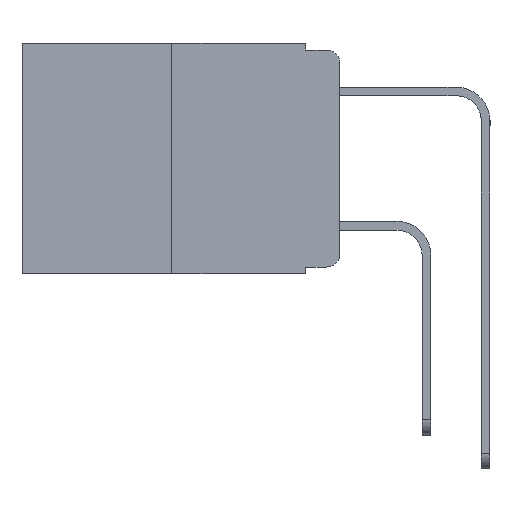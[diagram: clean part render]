
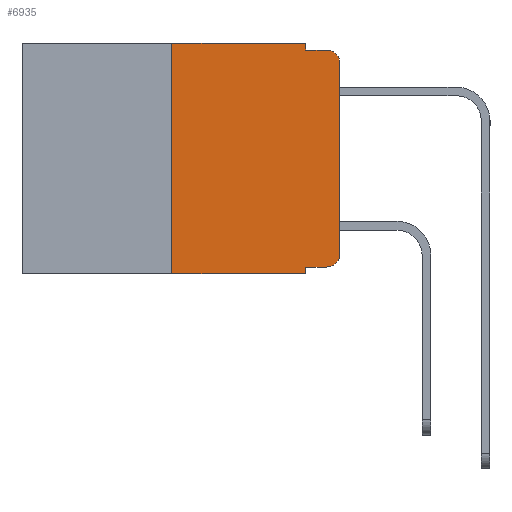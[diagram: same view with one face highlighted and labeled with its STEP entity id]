
A CAD part, left-side view. The second image highlights one B-rep face of the part: STEP entity #6935.
In plain terms, the highlighted planar face has unit normal (-1, 0, 0).
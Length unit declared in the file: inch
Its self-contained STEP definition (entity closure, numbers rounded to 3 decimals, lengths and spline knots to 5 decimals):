
#8 = FACE_OUTER_BOUND ( 'NONE', #3519, .T. ) ;
#575 = LINE ( 'NONE', #6948, #2765 ) ;
#703 = VECTOR ( 'NONE', #7074, 39.37008 ) ;
#1054 = CIRCLE ( 'NONE', #3146, 0.02 ) ;
#1242 = CARTESIAN_POINT ( 'NONE',  ( 0., 0.473, -0.343 ) ) ;
#1650 = CARTESIAN_POINT ( 'NONE',  ( 0., 0.02, -0.333 ) ) ;
#1763 = DIRECTION ( 'NONE',  ( 0., -1., 0. ) ) ;
#1765 = DIRECTION ( 'NONE',  ( 0., 0., 1. ) ) ;
#1862 = LINE ( 'NONE', #2055, #4319 ) ;
#2035 = VERTEX_POINT ( 'NONE', #3989 ) ;
#2053 = CARTESIAN_POINT ( 'NONE',  ( 0., 0.051, -0.333 ) ) ;
#2055 = CARTESIAN_POINT ( 'NONE',  ( 0., 0.051, 0. ) ) ;
#2287 = ORIENTED_EDGE ( 'NONE', *, *, #8767, .F. ) ;
#2603 = EDGE_CURVE ( 'NONE', #3111, #4419, #6063, .T. ) ;
#2765 = VECTOR ( 'NONE', #3821, 39.37008 ) ;
#2806 = ORIENTED_EDGE ( 'NONE', *, *, #2603, .T. ) ;
#2882 = CARTESIAN_POINT ( 'NONE',  ( 0., 0.02, -0.01 ) ) ;
#2961 = CARTESIAN_POINT ( 'NONE',  ( 0., 0.25, 0. ) ) ;
#3032 = DIRECTION ( 'NONE',  ( 0., -1., 0. ) ) ;
#3111 = VERTEX_POINT ( 'NONE', #1650 ) ;
#3146 = AXIS2_PLACEMENT_3D ( 'NONE', #10799, #4882, #11763 ) ;
#3317 = EDGE_CURVE ( 'NONE', #5770, #3111, #3462, .T. ) ;
#3462 = LINE ( 'NONE', #2053, #8555 ) ;
#3519 = EDGE_LOOP ( 'NONE', ( #10459, #9419, #2287, #11503, #12666, #12368, #8058, #8974, #6822, #2806 ) ) ;
#3821 = DIRECTION ( 'NONE',  ( 0., -1., 0. ) ) ;
#3989 = CARTESIAN_POINT ( 'NONE',  ( 0., 0., -0.03 ) ) ;
#4093 = CARTESIAN_POINT ( 'NONE',  ( 0., 0.051, -0.01 ) ) ;
#4191 = EDGE_CURVE ( 'NONE', #12171, #9761, #7765, .T. ) ;
#4319 = VECTOR ( 'NONE', #12962, 39.37008 ) ;
#4419 = VERTEX_POINT ( 'NONE', #6970 ) ;
#4425 = PLANE ( 'NONE',  #4759 ) ;
#4682 = CARTESIAN_POINT ( 'NONE',  ( 0., 0.051, -0.333 ) ) ;
#4699 = EDGE_CURVE ( 'NONE', #5770, #9761, #8820, .T. ) ;
#4759 = AXIS2_PLACEMENT_3D ( 'NONE', #11334, #5464, #12274 ) ;
#4882 = DIRECTION ( 'NONE',  ( -1., 0., 0. ) ) ;
#5383 = EDGE_CURVE ( 'NONE', #12171, #12336, #6310, .T. ) ;
#5464 = DIRECTION ( 'NONE',  ( 1., 0., 0. ) ) ;
#5770 = VERTEX_POINT ( 'NONE', #4682 ) ;
#6063 = CIRCLE ( 'NONE', #12346, 0.02 ) ;
#6310 = LINE ( 'NONE', #2961, #703 ) ;
#6785 = EDGE_CURVE ( 'NONE', #10905, #12877, #1862, .T. ) ;
#6822 = ORIENTED_EDGE ( 'NONE', *, *, #3317, .T. ) ;
#6844 = CARTESIAN_POINT ( 'NONE',  ( 0., 0.051, 0. ) ) ;
#6906 = CARTESIAN_POINT ( 'NONE',  ( 0., 0.473, 0. ) ) ;
#6935 = ADVANCED_FACE ( 'NONE', ( #8 ), #4425, .F. ) ;
#6948 = CARTESIAN_POINT ( 'NONE',  ( 0., 0.051, -0.01 ) ) ;
#6961 = CARTESIAN_POINT ( 'NONE',  ( 0., 0., 0. ) ) ;
#6970 = CARTESIAN_POINT ( 'NONE',  ( 0., 0., -0.313 ) ) ;
#7074 = DIRECTION ( 'NONE',  ( 0., 0., 1. ) ) ;
#7094 = LINE ( 'NONE', #6961, #7417 ) ;
#7115 = EDGE_CURVE ( 'NONE', #12336, #10905, #11371, .T. ) ;
#7417 = VECTOR ( 'NONE', #1765, 39.37008 ) ;
#7456 = VECTOR ( 'NONE', #1763, 39.37008 ) ;
#7581 = CARTESIAN_POINT ( 'NONE',  ( 0., 0.051, -0.343 ) ) ;
#7658 = CARTESIAN_POINT ( 'NONE',  ( 0., 0.25, 0. ) ) ;
#7765 = LINE ( 'NONE', #1242, #7456 ) ;
#8058 = ORIENTED_EDGE ( 'NONE', *, *, #4191, .T. ) ;
#8555 = VECTOR ( 'NONE', #3032, 39.37008 ) ;
#8767 = EDGE_CURVE ( 'NONE', #12877, #10045, #575, .T. ) ;
#8820 = LINE ( 'NONE', #6844, #11034 ) ;
#8849 = VECTOR ( 'NONE', #10782, 39.37008 ) ;
#8974 = ORIENTED_EDGE ( 'NONE', *, *, #4699, .F. ) ;
#9007 = DIRECTION ( 'NONE',  ( 0., 0., -1. ) ) ;
#9272 = CARTESIAN_POINT ( 'NONE',  ( 0., 0.02, -0.313 ) ) ;
#9388 = EDGE_CURVE ( 'NONE', #2035, #10045, #1054, .T. ) ;
#9419 = ORIENTED_EDGE ( 'NONE', *, *, #9388, .T. ) ;
#9761 = VERTEX_POINT ( 'NONE', #7581 ) ;
#10019 = EDGE_CURVE ( 'NONE', #4419, #2035, #7094, .T. ) ;
#10045 = VERTEX_POINT ( 'NONE', #2882 ) ;
#10238 = CARTESIAN_POINT ( 'NONE',  ( 0., 0.25, -0.343 ) ) ;
#10459 = ORIENTED_EDGE ( 'NONE', *, *, #10019, .T. ) ;
#10659 = DIRECTION ( 'NONE',  ( -1., 0., 0. ) ) ;
#10682 = DIRECTION ( 'NONE',  ( 0., 0., -1. ) ) ;
#10782 = DIRECTION ( 'NONE',  ( 0., -1., 0. ) ) ;
#10799 = CARTESIAN_POINT ( 'NONE',  ( 0., 0.02, -0.03 ) ) ;
#10905 = VERTEX_POINT ( 'NONE', #11178 ) ;
#11034 = VECTOR ( 'NONE', #10682, 39.37008 ) ;
#11178 = CARTESIAN_POINT ( 'NONE',  ( 0., 0.051, 0. ) ) ;
#11334 = CARTESIAN_POINT ( 'NONE',  ( 0., 0.473, 0. ) ) ;
#11371 = LINE ( 'NONE', #6906, #8849 ) ;
#11503 = ORIENTED_EDGE ( 'NONE', *, *, #6785, .F. ) ;
#11763 = DIRECTION ( 'NONE',  ( 0., 0., -1. ) ) ;
#12171 = VERTEX_POINT ( 'NONE', #10238 ) ;
#12274 = DIRECTION ( 'NONE',  ( 0., 0., -1. ) ) ;
#12336 = VERTEX_POINT ( 'NONE', #7658 ) ;
#12346 = AXIS2_PLACEMENT_3D ( 'NONE', #9272, #10659, #9007 ) ;
#12368 = ORIENTED_EDGE ( 'NONE', *, *, #5383, .F. ) ;
#12666 = ORIENTED_EDGE ( 'NONE', *, *, #7115, .F. ) ;
#12877 = VERTEX_POINT ( 'NONE', #4093 ) ;
#12962 = DIRECTION ( 'NONE',  ( 0., 0., -1. ) ) ;
